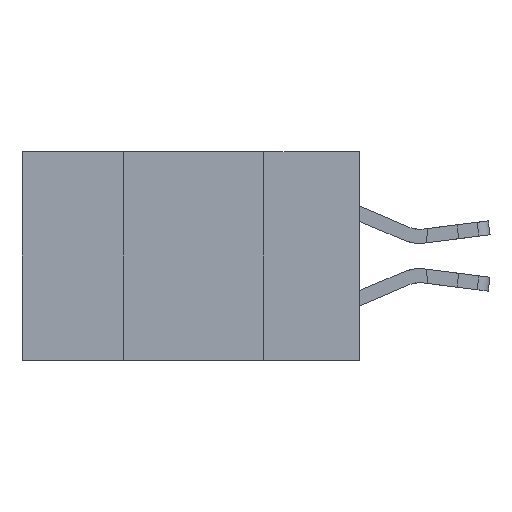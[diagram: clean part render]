
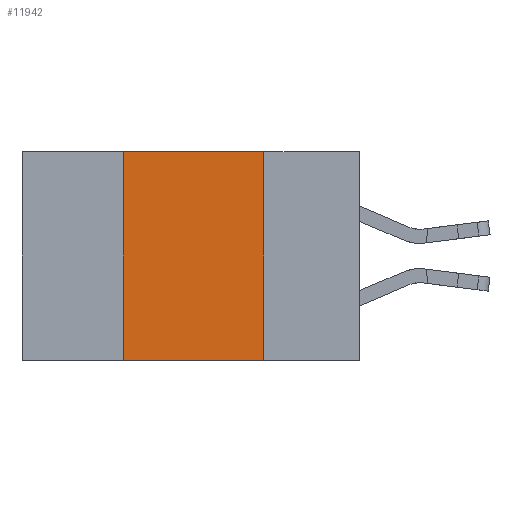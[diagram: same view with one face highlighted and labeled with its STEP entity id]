
A CAD part, left-side view. The second image highlights one B-rep face of the part: STEP entity #11942.
In plain terms, the highlighted planar face has unit normal (-1, 0, 0).
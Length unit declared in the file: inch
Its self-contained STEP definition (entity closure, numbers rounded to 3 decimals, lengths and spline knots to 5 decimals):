
#283 = ORIENTED_EDGE ( 'NONE', *, *, #21012, .T. ) ;
#1433 = CARTESIAN_POINT ( 'NONE',  ( 0., 0.42, -0.37 ) ) ;
#1947 = VERTEX_POINT ( 'NONE', #17049 ) ;
#2034 = CARTESIAN_POINT ( 'NONE',  ( 0., 0.17, -0.37 ) ) ;
#2210 = DIRECTION ( 'NONE',  ( 1., 0., 0. ) ) ;
#2217 = LINE ( 'NONE', #11011, #8767 ) ;
#2756 = DIRECTION ( 'NONE',  ( 0., 0., -1. ) ) ;
#3162 = CARTESIAN_POINT ( 'NONE',  ( 0., 0.6, 0. ) ) ;
#4628 = AXIS2_PLACEMENT_3D ( 'NONE', #20752, #2210, #20900 ) ;
#5105 = ORIENTED_EDGE ( 'NONE', *, *, #8107, .F. ) ;
#5937 = LINE ( 'NONE', #7282, #14342 ) ;
#6350 = VERTEX_POINT ( 'NONE', #16362 ) ;
#7056 = LINE ( 'NONE', #3162, #20960 ) ;
#7282 = CARTESIAN_POINT ( 'NONE',  ( 0., 0.6, -0.37 ) ) ;
#7951 = ORIENTED_EDGE ( 'NONE', *, *, #14534, .F. ) ;
#8107 = EDGE_CURVE ( 'NONE', #6350, #1947, #7056, .T. ) ;
#8767 = VECTOR ( 'NONE', #21135, 39.37008 ) ;
#9832 = VERTEX_POINT ( 'NONE', #2034 ) ;
#9973 = EDGE_CURVE ( 'NONE', #21427, #6350, #2217, .T. ) ;
#11011 = CARTESIAN_POINT ( 'NONE',  ( 0., 0.42, 0. ) ) ;
#11268 = CARTESIAN_POINT ( 'NONE',  ( 0., 0.17, 0. ) ) ;
#11942 = ADVANCED_FACE ( 'NONE', ( #18432 ), #12432, .F. ) ;
#12432 = PLANE ( 'NONE',  #4628 ) ;
#12743 = ORIENTED_EDGE ( 'NONE', *, *, #9973, .F. ) ;
#13288 = DIRECTION ( 'NONE',  ( 0., -1., 0. ) ) ;
#14342 = VECTOR ( 'NONE', #20457, 39.37008 ) ;
#14534 = EDGE_CURVE ( 'NONE', #1947, #9832, #19366, .T. ) ;
#16362 = CARTESIAN_POINT ( 'NONE',  ( 0., 0.42, 0. ) ) ;
#17049 = CARTESIAN_POINT ( 'NONE',  ( 0., 0.17, 0. ) ) ;
#18432 = FACE_OUTER_BOUND ( 'NONE', #20869, .T. ) ;
#19105 = VECTOR ( 'NONE', #2756, 39.37008 ) ;
#19366 = LINE ( 'NONE', #11268, #19105 ) ;
#20457 = DIRECTION ( 'NONE',  ( 0., -1., 0. ) ) ;
#20752 = CARTESIAN_POINT ( 'NONE',  ( 0., 0.6, 0. ) ) ;
#20869 = EDGE_LOOP ( 'NONE', ( #7951, #5105, #12743, #283 ) ) ;
#20900 = DIRECTION ( 'NONE',  ( 0., 0., -1. ) ) ;
#20960 = VECTOR ( 'NONE', #13288, 39.37008 ) ;
#21012 = EDGE_CURVE ( 'NONE', #21427, #9832, #5937, .T. ) ;
#21135 = DIRECTION ( 'NONE',  ( 0., 0., 1. ) ) ;
#21427 = VERTEX_POINT ( 'NONE', #1433 ) ;
